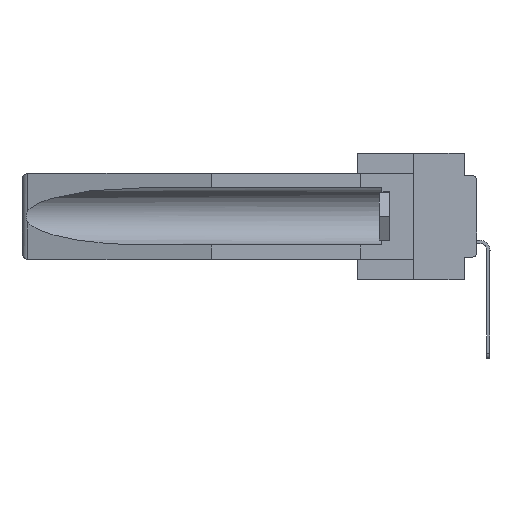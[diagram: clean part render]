
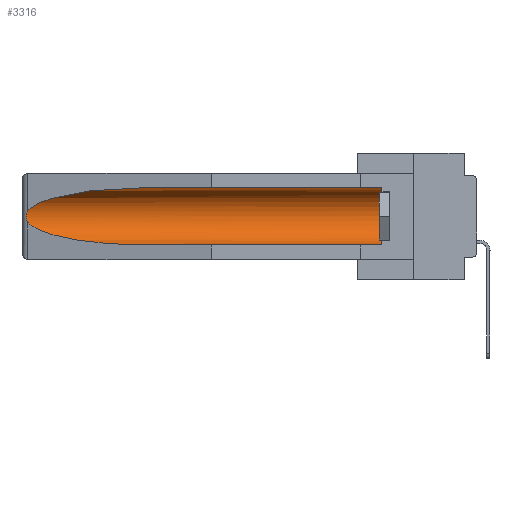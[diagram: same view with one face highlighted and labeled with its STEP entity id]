
A CAD part, left-side view. The second image highlights one B-rep face of the part: STEP entity #3316.
In plain terms, the highlighted cylindrical face has radius 2.857 mm (diameter 5.715 mm), a partial arc.
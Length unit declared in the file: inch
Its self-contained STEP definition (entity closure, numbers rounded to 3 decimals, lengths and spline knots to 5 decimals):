
#406 = EDGE_CURVE ( 'NONE', #15244, #15200, #8443, .T. ) ;
#1018 = DIRECTION ( 'NONE',  ( 0., 1., 0. ) ) ;
#1804 = CARTESIAN_POINT ( 'NONE',  ( 0.26654, 1.53092, -0.15636 ) ) ;
#2426 = AXIS2_PLACEMENT_3D ( 'NONE', #26113, #18030, #5739 ) ;
#3316 = ADVANCED_FACE ( 'NONE', ( #22552 ), #17843, .F. ) ;
#3556 = EDGE_LOOP ( 'NONE', ( #30624, #17593, #29444, #26395, #25983, #10429 ) ) ;
#3891 = CARTESIAN_POINT ( 'NONE',  ( 0.155, -0.30754, -0.059 ) ) ;
#3941 = CARTESIAN_POINT ( 'NONE',  ( 0.155, 1.07973, -0.284 ) ) ;
#4241 = CARTESIAN_POINT ( 'NONE',  ( 0.26537, 1.52718, -0.14972 ) ) ;
#4268 = CARTESIAN_POINT ( 'NONE',  ( 0.21114, 1.30732, -0.284 ) ) ;
#4394 = CARTESIAN_POINT ( 'NONE',  ( 0.2675, 1.53308, -0.16763 ) ) ;
#5643 = EDGE_CURVE ( 'NONE', #16920, #14889, #5845, .T. ) ;
#5739 = DIRECTION ( 'NONE',  ( 0., 0., 1. ) ) ;
#5845 =( BOUNDED_CURVE ( )  B_SPLINE_CURVE ( 3, ( #30623, #25480, #8473, #28204 ),
 .UNSPECIFIED., .F., .F. ) 
 B_SPLINE_CURVE_WITH_KNOTS ( ( 4, 4 ),
 ( 4.71239, 6.08839 ),
 .UNSPECIFIED. ) 
 CURVE ( )  GEOMETRIC_REPRESENTATION_ITEM ( )  RATIONAL_B_SPLINE_CURVE ( ( 1., 0.848, 0.848, 1. ) ) 
 REPRESENTATION_ITEM ( '' )  );
#6817 = VERTEX_POINT ( 'NONE', #28372 ) ;
#6822 = CARTESIAN_POINT ( 'NONE',  ( 0.26655, 1.53094, -0.18657 ) ) ;
#7237 = CARTESIAN_POINT ( 'NONE',  ( 0.155, 1.07973, -0.059 ) ) ;
#7832 = CARTESIAN_POINT ( 'NONE',  ( 0.155, -0.30754, -0.1715 ) ) ;
#8443 = LINE ( 'NONE', #10694, #26578 ) ;
#8473 = CARTESIAN_POINT ( 'NONE',  ( 0.25451, 1.48313, -0.09465 ) ) ;
#8627 = CARTESIAN_POINT ( 'NONE',  ( 0.25451, 1.48313, -0.24835 ) ) ;
#8761 = CARTESIAN_POINT ( 'NONE',  ( 0.26597, 1.5296, -0.19026 ) ) ;
#10429 = ORIENTED_EDGE ( 'NONE', *, *, #19264, .T. ) ;
#10694 = CARTESIAN_POINT ( 'NONE',  ( 0.155, -0.30754, -0.284 ) ) ;
#14250 = CARTESIAN_POINT ( 'NONE',  ( 0.2673, 1.5327, -0.16383 ) ) ;
#14889 = VERTEX_POINT ( 'NONE', #23266 ) ;
#15200 = VERTEX_POINT ( 'NONE', #25649 ) ;
#15244 = VERTEX_POINT ( 'NONE', #30804 ) ;
#16039 = CARTESIAN_POINT ( 'NONE',  ( 0.26597, 1.52961, -0.15275 ) ) ;
#16920 = VERTEX_POINT ( 'NONE', #7237 ) ;
#17593 = ORIENTED_EDGE ( 'NONE', *, *, #22905, .T. ) ;
#17843 = CYLINDRICAL_SURFACE ( 'NONE', #25611, 0.1125 ) ;
#18030 = DIRECTION ( 'NONE',  ( 0., -1., 0. ) ) ;
#18440 = DIRECTION ( 'NONE',  ( 0., 1., 0. ) ) ;
#18619 = CARTESIAN_POINT ( 'NONE',  ( 0.2675, 1.53308, -0.17534 ) ) ;
#18780 = CARTESIAN_POINT ( 'NONE',  ( 0.26537, 1.52718, -0.19328 ) ) ;
#19264 = EDGE_CURVE ( 'NONE', #6817, #16920, #25897, .T. ) ;
#20901 = DIRECTION ( 'NONE',  ( 0., 1., 0. ) ) ;
#21177 = EDGE_CURVE ( 'NONE', #22972, #15200, #30210, .T. ) ;
#21566 = B_SPLINE_CURVE_WITH_KNOTS ( 'NONE', 3,
 ( #4241, #16039, #1804, #14250, #4394, #18619, #25919, #6822, #8761, #18780 ),
 .UNSPECIFIED., .F., .F.,
 ( 4, 2, 2, 2, 4 ),
 ( 0., 0.00029, 0.00058, 0.00087, 0.00117 ),
 .UNSPECIFIED. ) ;
#22552 = FACE_OUTER_BOUND ( 'NONE', #3556, .T. ) ;
#22905 = EDGE_CURVE ( 'NONE', #14889, #22972, #21566, .T. ) ;
#22972 = VERTEX_POINT ( 'NONE', #28968 ) ;
#23266 = CARTESIAN_POINT ( 'NONE',  ( 0.26537, 1.52718, -0.14972 ) ) ;
#23304 = VECTOR ( 'NONE', #18440, 39.37008 ) ;
#23571 = CIRCLE ( 'NONE', #2426, 0.1125 ) ;
#25480 = CARTESIAN_POINT ( 'NONE',  ( 0.21114, 1.30732, -0.059 ) ) ;
#25611 = AXIS2_PLACEMENT_3D ( 'NONE', #7832, #1018, #30284 ) ;
#25649 = CARTESIAN_POINT ( 'NONE',  ( 0.155, 1.07973, -0.284 ) ) ;
#25813 = EDGE_CURVE ( 'NONE', #15244, #6817, #23571, .T. ) ;
#25897 = LINE ( 'NONE', #3891, #23304 ) ;
#25919 = CARTESIAN_POINT ( 'NONE',  ( 0.2673, 1.53269, -0.17917 ) ) ;
#25983 = ORIENTED_EDGE ( 'NONE', *, *, #25813, .T. ) ;
#26109 = CARTESIAN_POINT ( 'NONE',  ( 0.26537, 1.52718, -0.19328 ) ) ;
#26113 = CARTESIAN_POINT ( 'NONE',  ( 0.155, 0.126, -0.1715 ) ) ;
#26395 = ORIENTED_EDGE ( 'NONE', *, *, #406, .F. ) ;
#26578 = VECTOR ( 'NONE', #20901, 39.37008 ) ;
#28204 = CARTESIAN_POINT ( 'NONE',  ( 0.26537, 1.52718, -0.14972 ) ) ;
#28372 = CARTESIAN_POINT ( 'NONE',  ( 0.155, 0.126, -0.059 ) ) ;
#28968 = CARTESIAN_POINT ( 'NONE',  ( 0.26537, 1.52718, -0.19328 ) ) ;
#29444 = ORIENTED_EDGE ( 'NONE', *, *, #21177, .T. ) ;
#30210 =( BOUNDED_CURVE ( )  B_SPLINE_CURVE ( 3, ( #26109, #8627, #4268, #3941 ),
 .UNSPECIFIED., .F., .F. ) 
 B_SPLINE_CURVE_WITH_KNOTS ( ( 4, 4 ),
 ( 0.1948, 1.5708 ),
 .UNSPECIFIED. ) 
 CURVE ( )  GEOMETRIC_REPRESENTATION_ITEM ( )  RATIONAL_B_SPLINE_CURVE ( ( 1., 0.848, 0.848, 1. ) ) 
 REPRESENTATION_ITEM ( '' )  );
#30284 = DIRECTION ( 'NONE',  ( 0., 0., 1. ) ) ;
#30623 = CARTESIAN_POINT ( 'NONE',  ( 0.155, 1.07973, -0.059 ) ) ;
#30624 = ORIENTED_EDGE ( 'NONE', *, *, #5643, .T. ) ;
#30804 = CARTESIAN_POINT ( 'NONE',  ( 0.155, 0.126, -0.284 ) ) ;
